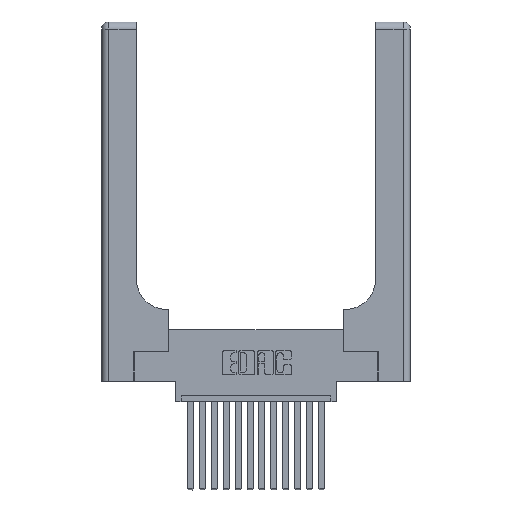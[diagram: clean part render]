
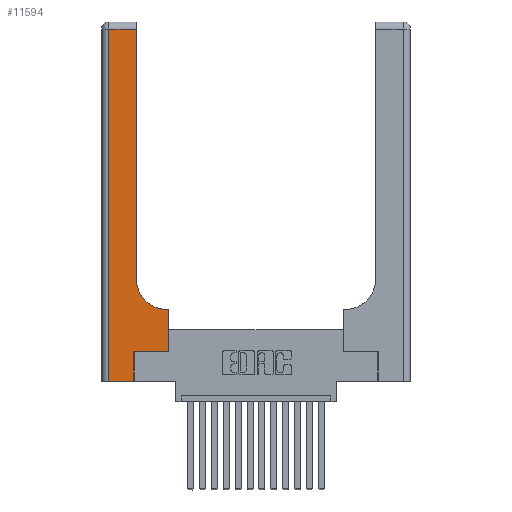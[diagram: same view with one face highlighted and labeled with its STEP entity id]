
A CAD part, top view. The second image highlights one B-rep face of the part: STEP entity #11594.
In plain terms, the highlighted planar face has unit normal (0, 0, 1).
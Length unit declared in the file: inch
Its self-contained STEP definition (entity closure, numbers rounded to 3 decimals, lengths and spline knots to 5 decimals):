
#4 = VERTEX_POINT ( 'NONE', #14542 ) ;
#51 = CARTESIAN_POINT ( 'NONE',  ( 0.269, 0., 0.37 ) ) ;
#134 = DIRECTION ( 'NONE',  ( 0., 0., -1. ) ) ;
#481 = ORIENTED_EDGE ( 'NONE', *, *, #8674, .T. ) ;
#879 = EDGE_CURVE ( 'NONE', #4, #16045, #14365, .T. ) ;
#1317 = ORIENTED_EDGE ( 'NONE', *, *, #879, .T. ) ;
#1700 = ORIENTED_EDGE ( 'NONE', *, *, #6052, .T. ) ;
#1709 = LINE ( 'NONE', #4578, #18222 ) ;
#1719 = AXIS2_PLACEMENT_3D ( 'NONE', #12568, #134, #16863 ) ;
#1924 = EDGE_LOOP ( 'NONE', ( #17644, #6422, #13638, #481, #13307, #1700, #1317, #4194, #2768 ) ) ;
#2537 = CIRCLE ( 'NONE', #6663, 0.25 ) ;
#2639 = EDGE_CURVE ( 'NONE', #13334, #3520, #10794, .T. ) ;
#2768 = ORIENTED_EDGE ( 'NONE', *, *, #12559, .T. ) ;
#2818 = DIRECTION ( 'NONE',  ( -1., 0., 0. ) ) ;
#2891 = CARTESIAN_POINT ( 'NONE',  ( 0.2915, 0.85, 0.37 ) ) ;
#2935 = CARTESIAN_POINT ( 'NONE',  ( 0.269, 0., 0.37 ) ) ;
#3096 = DIRECTION ( 'NONE',  ( 1., 0., 0. ) ) ;
#3189 = LINE ( 'NONE', #51, #15283 ) ;
#3520 = VERTEX_POINT ( 'NONE', #12216 ) ;
#3703 = CARTESIAN_POINT ( 'NONE',  ( 0.5585, 0.25, 0.37 ) ) ;
#3983 = CARTESIAN_POINT ( 'NONE',  ( 0.5415, 0.85, 0.37 ) ) ;
#4194 = ORIENTED_EDGE ( 'NONE', *, *, #6529, .T. ) ;
#4250 = CARTESIAN_POINT ( 'NONE',  ( 0.2915, 3., 0.37 ) ) ;
#4578 = CARTESIAN_POINT ( 'NONE',  ( 0., 0., 0.37 ) ) ;
#4677 = CARTESIAN_POINT ( 'NONE',  ( 0.269, 0.25, 0.37 ) ) ;
#4761 = EDGE_CURVE ( 'NONE', #10864, #5943, #12930, .T. ) ;
#4989 = VERTEX_POINT ( 'NONE', #2935 ) ;
#5161 = VECTOR ( 'NONE', #16094, 39.37008 ) ;
#5897 = DIRECTION ( 'NONE',  ( 0., 1., 0. ) ) ;
#5943 = VERTEX_POINT ( 'NONE', #11735 ) ;
#5964 = VECTOR ( 'NONE', #5897, 39.37008 ) ;
#6052 = EDGE_CURVE ( 'NONE', #11230, #4, #17291, .T. ) ;
#6238 = DIRECTION ( 'NONE',  ( -1., 0., 0. ) ) ;
#6422 = ORIENTED_EDGE ( 'NONE', *, *, #13851, .T. ) ;
#6529 = EDGE_CURVE ( 'NONE', #16045, #16913, #14624, .T. ) ;
#6663 = AXIS2_PLACEMENT_3D ( 'NONE', #3983, #9672, #15271 ) ;
#7757 = CARTESIAN_POINT ( 'NONE',  ( 0.5415, 0.6, 0.37 ) ) ;
#8389 = PLANE ( 'NONE',  #1719 ) ;
#8600 = DIRECTION ( 'NONE',  ( 0., 1., 0. ) ) ;
#8674 = EDGE_CURVE ( 'NONE', #5943, #4989, #1709, .T. ) ;
#8873 = VECTOR ( 'NONE', #2818, 39.37008 ) ;
#8927 = FACE_OUTER_BOUND ( 'NONE', #1924, .T. ) ;
#8960 = DIRECTION ( 'NONE',  ( 1., 0., 0. ) ) ;
#9021 = CARTESIAN_POINT ( 'NONE',  ( 0.269, 0.25, 0.37 ) ) ;
#9672 = DIRECTION ( 'NONE',  ( 0., 0., -1. ) ) ;
#9760 = CARTESIAN_POINT ( 'NONE',  ( 0.5585, 0.6, 0.37 ) ) ;
#9873 = CARTESIAN_POINT ( 'NONE',  ( 0., 2.94, 0.37 ) ) ;
#10030 = VECTOR ( 'NONE', #8960, 39.37008 ) ;
#10794 = LINE ( 'NONE', #4250, #5964 ) ;
#10864 = VERTEX_POINT ( 'NONE', #17575 ) ;
#10887 = VECTOR ( 'NONE', #6238, 39.37008 ) ;
#11230 = VERTEX_POINT ( 'NONE', #4677 ) ;
#11360 = CARTESIAN_POINT ( 'NONE',  ( 0.06, 3., 0.37 ) ) ;
#11594 = ADVANCED_FACE ( 'NONE', ( #8927 ), #8389, .F. ) ;
#11735 = CARTESIAN_POINT ( 'NONE',  ( 0.06, 0., 0.37 ) ) ;
#12216 = CARTESIAN_POINT ( 'NONE',  ( 0.2915, 2.94, 0.37 ) ) ;
#12327 = EDGE_CURVE ( 'NONE', #4989, #11230, #3189, .T. ) ;
#12559 = EDGE_CURVE ( 'NONE', #16913, #13334, #2537, .T. ) ;
#12568 = CARTESIAN_POINT ( 'NONE',  ( 0., 3., 0.37 ) ) ;
#12888 = DIRECTION ( 'NONE',  ( 0., -1., 0. ) ) ;
#12930 = LINE ( 'NONE', #11360, #13157 ) ;
#13157 = VECTOR ( 'NONE', #12888, 39.37008 ) ;
#13307 = ORIENTED_EDGE ( 'NONE', *, *, #12327, .T. ) ;
#13334 = VERTEX_POINT ( 'NONE', #2891 ) ;
#13638 = ORIENTED_EDGE ( 'NONE', *, *, #4761, .T. ) ;
#13851 = EDGE_CURVE ( 'NONE', #3520, #10864, #14585, .T. ) ;
#14365 = LINE ( 'NONE', #3703, #5161 ) ;
#14542 = CARTESIAN_POINT ( 'NONE',  ( 0.5585, 0.25, 0.37 ) ) ;
#14585 = LINE ( 'NONE', #9873, #8873 ) ;
#14624 = LINE ( 'NONE', #15827, #10887 ) ;
#15271 = DIRECTION ( 'NONE',  ( 1., 0., 0. ) ) ;
#15283 = VECTOR ( 'NONE', #8600, 39.37008 ) ;
#15827 = CARTESIAN_POINT ( 'NONE',  ( 0.2915, 0.6, 0.37 ) ) ;
#16045 = VERTEX_POINT ( 'NONE', #9760 ) ;
#16094 = DIRECTION ( 'NONE',  ( 0., 1., 0. ) ) ;
#16863 = DIRECTION ( 'NONE',  ( -1., 0., 0. ) ) ;
#16913 = VERTEX_POINT ( 'NONE', #7757 ) ;
#17291 = LINE ( 'NONE', #9021, #10030 ) ;
#17575 = CARTESIAN_POINT ( 'NONE',  ( 0.06, 2.94, 0.37 ) ) ;
#17644 = ORIENTED_EDGE ( 'NONE', *, *, #2639, .T. ) ;
#18222 = VECTOR ( 'NONE', #3096, 39.37008 ) ;
